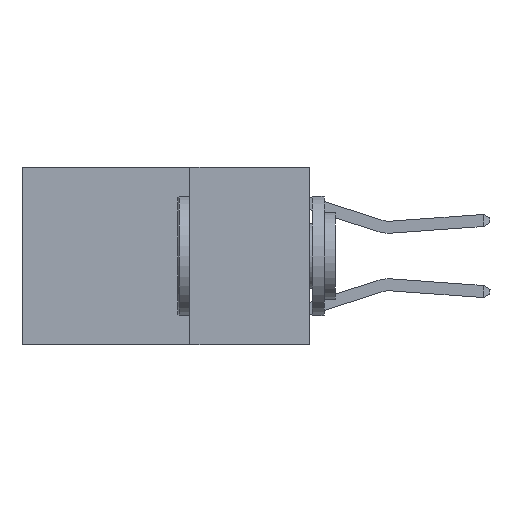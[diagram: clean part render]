
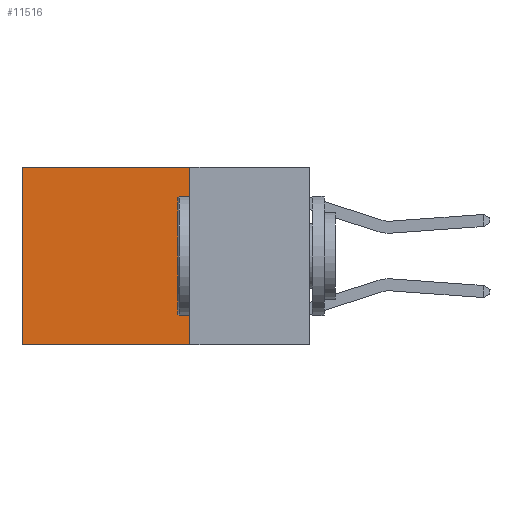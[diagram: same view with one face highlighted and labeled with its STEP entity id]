
A CAD part, left-side view. The second image highlights one B-rep face of the part: STEP entity #11516.
In plain terms, the highlighted planar face has unit normal (-1, 0, 0).
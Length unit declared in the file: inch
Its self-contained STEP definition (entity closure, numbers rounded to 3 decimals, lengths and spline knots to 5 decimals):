
#53 = PLANE ( 'NONE',  #8037 ) ;
#1577 = CARTESIAN_POINT ( 'NONE',  ( 0.2625, 0.25, 0. ) ) ;
#1622 = CARTESIAN_POINT ( 'NONE',  ( 0.2625, 0.25, 0. ) ) ;
#1947 = ORIENTED_EDGE ( 'NONE', *, *, #27088, .T. ) ;
#2411 = DIRECTION ( 'NONE',  ( 1., 0., 0. ) ) ;
#2648 = VECTOR ( 'NONE', #11585, 39.37008 ) ;
#3920 = EDGE_CURVE ( 'NONE', #21923, #7825, #8852, .T. ) ;
#4312 = ORIENTED_EDGE ( 'NONE', *, *, #3920, .T. ) ;
#6577 = VERTEX_POINT ( 'NONE', #24400 ) ;
#7825 = VERTEX_POINT ( 'NONE', #7862 ) ;
#7862 = CARTESIAN_POINT ( 'NONE',  ( 0.2625, 0.6, -0.37 ) ) ;
#8037 = AXIS2_PLACEMENT_3D ( 'NONE', #16324, #2411, #18613 ) ;
#8385 = VECTOR ( 'NONE', #18447, 39.37008 ) ;
#8825 = EDGE_LOOP ( 'NONE', ( #4312, #28916, #15293, #1947 ) ) ;
#8852 = LINE ( 'NONE', #23009, #2648 ) ;
#11516 = ADVANCED_FACE ( 'NONE', ( #22769 ), #53, .F. ) ;
#11585 = DIRECTION ( 'NONE',  ( 0., 0., -1. ) ) ;
#14578 = EDGE_CURVE ( 'NONE', #6577, #23300, #23670, .T. ) ;
#15293 = ORIENTED_EDGE ( 'NONE', *, *, #14578, .F. ) ;
#15519 = DIRECTION ( 'NONE',  ( 0., 0., -1. ) ) ;
#16324 = CARTESIAN_POINT ( 'NONE',  ( 0.2625, 0.25, 0. ) ) ;
#16904 = VECTOR ( 'NONE', #15519, 39.37008 ) ;
#17835 = DIRECTION ( 'NONE',  ( 0., 1., 0. ) ) ;
#18447 = DIRECTION ( 'NONE',  ( 0., 1., 0. ) ) ;
#18613 = DIRECTION ( 'NONE',  ( 0., 0., -1. ) ) ;
#20381 = EDGE_CURVE ( 'NONE', #23300, #7825, #21347, .T. ) ;
#20614 = CARTESIAN_POINT ( 'NONE',  ( 0.2625, 0.25, -0.37 ) ) ;
#21347 = LINE ( 'NONE', #20614, #8385 ) ;
#21475 = LINE ( 'NONE', #1622, #22190 ) ;
#21923 = VERTEX_POINT ( 'NONE', #28171 ) ;
#22190 = VECTOR ( 'NONE', #17835, 39.37008 ) ;
#22769 = FACE_OUTER_BOUND ( 'NONE', #8825, .T. ) ;
#23009 = CARTESIAN_POINT ( 'NONE',  ( 0.2625, 0.6, 0. ) ) ;
#23300 = VERTEX_POINT ( 'NONE', #26141 ) ;
#23670 = LINE ( 'NONE', #1577, #16904 ) ;
#24400 = CARTESIAN_POINT ( 'NONE',  ( 0.2625, 0.25, 0. ) ) ;
#26141 = CARTESIAN_POINT ( 'NONE',  ( 0.2625, 0.25, -0.37 ) ) ;
#27088 = EDGE_CURVE ( 'NONE', #6577, #21923, #21475, .T. ) ;
#28171 = CARTESIAN_POINT ( 'NONE',  ( 0.2625, 0.6, 0. ) ) ;
#28916 = ORIENTED_EDGE ( 'NONE', *, *, #20381, .F. ) ;
